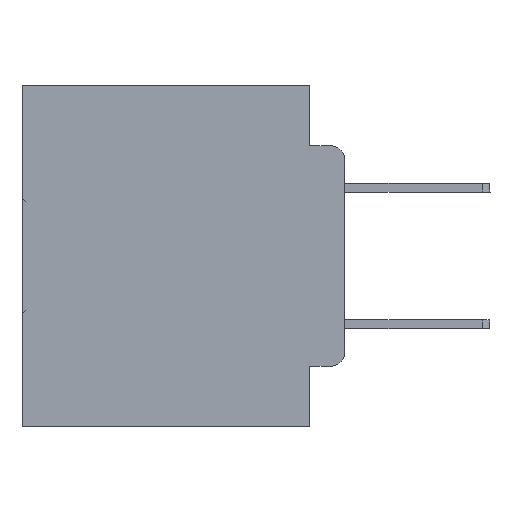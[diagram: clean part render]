
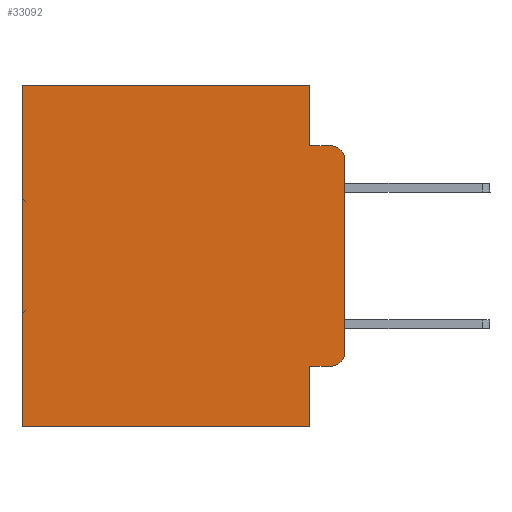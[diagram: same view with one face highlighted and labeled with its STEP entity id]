
A CAD part, left-side view. The second image highlights one B-rep face of the part: STEP entity #33092.
In plain terms, the highlighted planar face has unit normal (-1, 0, 0).
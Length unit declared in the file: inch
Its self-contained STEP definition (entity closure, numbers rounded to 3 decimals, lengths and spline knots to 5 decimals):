
#588 = ORIENTED_EDGE ( 'NONE', *, *, #24651, .F. ) ;
#628 = CARTESIAN_POINT ( 'NONE',  ( 0.298, 0.051, -0.0885 ) ) ;
#731 = VECTOR ( 'NONE', #33397, 39.37008 ) ;
#907 = CARTESIAN_POINT ( 'NONE',  ( 0.298, 0.051, -0.5 ) ) ;
#955 = VECTOR ( 'NONE', #11180, 39.37008 ) ;
#1056 = VERTEX_POINT ( 'NONE', #26771 ) ;
#1478 = ORIENTED_EDGE ( 'NONE', *, *, #9771, .F. ) ;
#1642 = LINE ( 'NONE', #12152, #17970 ) ;
#1877 = DIRECTION ( 'NONE',  ( 0., 0., -1. ) ) ;
#1917 = DIRECTION ( 'NONE',  ( -1., 0., 0. ) ) ;
#2697 = VERTEX_POINT ( 'NONE', #628 ) ;
#2842 = ORIENTED_EDGE ( 'NONE', *, *, #16066, .T. ) ;
#3617 = DIRECTION ( 'NONE',  ( 0., 1., 0. ) ) ;
#3706 = LINE ( 'NONE', #30054, #32607 ) ;
#5044 = EDGE_CURVE ( 'NONE', #20104, #5968, #7029, .T. ) ;
#5333 = ORIENTED_EDGE ( 'NONE', *, *, #15343, .T. ) ;
#5664 = CARTESIAN_POINT ( 'NONE',  ( 0.298, 0., 0. ) ) ;
#5682 = EDGE_LOOP ( 'NONE', ( #1478, #16547, #11442, #15047, #5333, #11505, #17799, #588, #2842, #17843 ) ) ;
#5896 = LINE ( 'NONE', #14200, #22973 ) ;
#5968 = VERTEX_POINT ( 'NONE', #30624 ) ;
#6327 = CARTESIAN_POINT ( 'NONE',  ( 0.298, 0.051, 0. ) ) ;
#6389 = AXIS2_PLACEMENT_3D ( 'NONE', #20344, #1917, #12433 ) ;
#7029 = LINE ( 'NONE', #7189, #15023 ) ;
#7189 = CARTESIAN_POINT ( 'NONE',  ( 0.298, 0.473, 0. ) ) ;
#7194 = FACE_OUTER_BOUND ( 'NONE', #5682, .T. ) ;
#7422 = VERTEX_POINT ( 'NONE', #15016 ) ;
#9586 = CARTESIAN_POINT ( 'NONE',  ( 0.298, 0.473, 0. ) ) ;
#9771 = EDGE_CURVE ( 'NONE', #31191, #25698, #22729, .T. ) ;
#10043 = EDGE_CURVE ( 'NONE', #26530, #2697, #19109, .T. ) ;
#10832 = LINE ( 'NONE', #13937, #955 ) ;
#11128 = DIRECTION ( 'NONE',  ( 0., 0., -1. ) ) ;
#11180 = DIRECTION ( 'NONE',  ( 0., 1., 0. ) ) ;
#11442 = ORIENTED_EDGE ( 'NONE', *, *, #29257, .F. ) ;
#11505 = ORIENTED_EDGE ( 'NONE', *, *, #5044, .T. ) ;
#12152 = CARTESIAN_POINT ( 'NONE',  ( 0.298, 0.051, -0.4115 ) ) ;
#12433 = DIRECTION ( 'NONE',  ( 0., 0., -1. ) ) ;
#13630 = VECTOR ( 'NONE', #3617, 39.37008 ) ;
#13655 = VERTEX_POINT ( 'NONE', #907 ) ;
#13937 = CARTESIAN_POINT ( 'NONE',  ( 0.298, 0., -0.5 ) ) ;
#14200 = CARTESIAN_POINT ( 'NONE',  ( 0.298, 0.051, -0.0885 ) ) ;
#15016 = CARTESIAN_POINT ( 'NONE',  ( 0.298, 0.02, -0.4115 ) ) ;
#15023 = VECTOR ( 'NONE', #28711, 39.37008 ) ;
#15047 = ORIENTED_EDGE ( 'NONE', *, *, #10043, .F. ) ;
#15154 = DIRECTION ( 'NONE',  ( 1., 0., 0. ) ) ;
#15343 = EDGE_CURVE ( 'NONE', #26530, #20104, #29978, .T. ) ;
#16066 = EDGE_CURVE ( 'NONE', #1056, #7422, #1642, .T. ) ;
#16547 = ORIENTED_EDGE ( 'NONE', *, *, #28855, .T. ) ;
#16946 = CARTESIAN_POINT ( 'NONE',  ( 0.298, 0., -0.1085 ) ) ;
#17799 = ORIENTED_EDGE ( 'NONE', *, *, #30270, .F. ) ;
#17843 = ORIENTED_EDGE ( 'NONE', *, *, #28152, .T. ) ;
#17970 = VECTOR ( 'NONE', #20062, 39.37008 ) ;
#18557 = CIRCLE ( 'NONE', #19647, 0.02 ) ;
#19109 = LINE ( 'NONE', #6327, #24336 ) ;
#19479 = CARTESIAN_POINT ( 'NONE',  ( 0.298, 0., -0.3915 ) ) ;
#19647 = AXIS2_PLACEMENT_3D ( 'NONE', #21797, #19738, #27481 ) ;
#19738 = DIRECTION ( 'NONE',  ( -1., 0., 0. ) ) ;
#20062 = DIRECTION ( 'NONE',  ( 0., -1., 0. ) ) ;
#20104 = VERTEX_POINT ( 'NONE', #9586 ) ;
#20344 = CARTESIAN_POINT ( 'NONE',  ( 0.298, 0.02, -0.3915 ) ) ;
#21797 = CARTESIAN_POINT ( 'NONE',  ( 0.298, 0.02, -0.1085 ) ) ;
#22729 = LINE ( 'NONE', #33560, #731 ) ;
#22973 = VECTOR ( 'NONE', #24699, 39.37008 ) ;
#24096 = DIRECTION ( 'NONE',  ( 0., 0., -1. ) ) ;
#24336 = VECTOR ( 'NONE', #24096, 39.37008 ) ;
#24450 = VERTEX_POINT ( 'NONE', #27550 ) ;
#24651 = EDGE_CURVE ( 'NONE', #1056, #13655, #3706, .T. ) ;
#24699 = DIRECTION ( 'NONE',  ( 0., -1., 0. ) ) ;
#24975 = CARTESIAN_POINT ( 'NONE',  ( 0.298, 0.051, 0. ) ) ;
#24976 = AXIS2_PLACEMENT_3D ( 'NONE', #28899, #15154, #1877 ) ;
#25698 = VERTEX_POINT ( 'NONE', #19479 ) ;
#26530 = VERTEX_POINT ( 'NONE', #24975 ) ;
#26771 = CARTESIAN_POINT ( 'NONE',  ( 0.298, 0.051, -0.4115 ) ) ;
#27481 = DIRECTION ( 'NONE',  ( 0., 0., -1. ) ) ;
#27550 = CARTESIAN_POINT ( 'NONE',  ( 0.298, 0.02, -0.0885 ) ) ;
#28152 = EDGE_CURVE ( 'NONE', #7422, #25698, #31679, .T. ) ;
#28221 = PLANE ( 'NONE',  #24976 ) ;
#28711 = DIRECTION ( 'NONE',  ( 0., 0., -1. ) ) ;
#28855 = EDGE_CURVE ( 'NONE', #31191, #24450, #18557, .T. ) ;
#28899 = CARTESIAN_POINT ( 'NONE',  ( 0.298, 0., 0. ) ) ;
#29257 = EDGE_CURVE ( 'NONE', #2697, #24450, #5896, .T. ) ;
#29978 = LINE ( 'NONE', #5664, #13630 ) ;
#30054 = CARTESIAN_POINT ( 'NONE',  ( 0.298, 0.051, 0. ) ) ;
#30270 = EDGE_CURVE ( 'NONE', #13655, #5968, #10832, .T. ) ;
#30624 = CARTESIAN_POINT ( 'NONE',  ( 0.298, 0.473, -0.5 ) ) ;
#31191 = VERTEX_POINT ( 'NONE', #16946 ) ;
#31679 = CIRCLE ( 'NONE', #6389, 0.02 ) ;
#32607 = VECTOR ( 'NONE', #11128, 39.37008 ) ;
#33092 = ADVANCED_FACE ( 'NONE', ( #7194 ), #28221, .F. ) ;
#33397 = DIRECTION ( 'NONE',  ( 0., 0., -1. ) ) ;
#33560 = CARTESIAN_POINT ( 'NONE',  ( 0.298, 0., 0. ) ) ;
